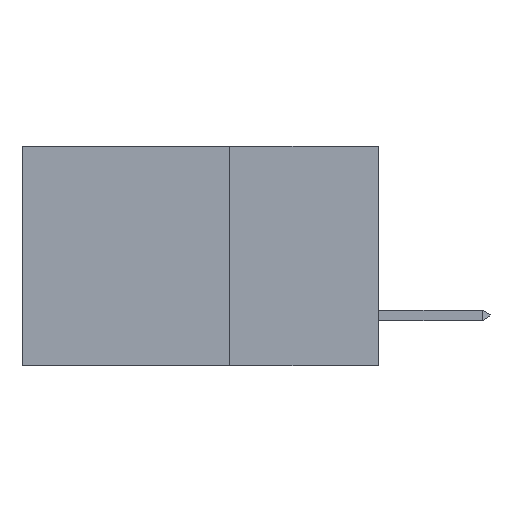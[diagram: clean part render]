
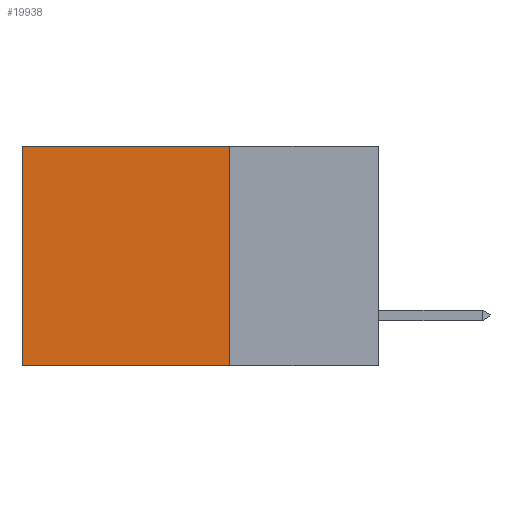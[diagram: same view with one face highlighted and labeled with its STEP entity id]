
A CAD part, left-side view. The second image highlights one B-rep face of the part: STEP entity #19938.
In plain terms, the highlighted planar face has unit normal (-1, 0, 0).
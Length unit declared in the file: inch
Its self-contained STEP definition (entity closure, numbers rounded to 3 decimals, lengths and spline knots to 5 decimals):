
#2656 = CARTESIAN_POINT ( 'NONE',  ( 0.2615, 0.25, -0.37 ) ) ;
#3022 = ORIENTED_EDGE ( 'NONE', *, *, #3099, .T. ) ;
#3099 = EDGE_CURVE ( 'NONE', #11433, #8185, #10697, .T. ) ;
#3180 = ORIENTED_EDGE ( 'NONE', *, *, #11354, .F. ) ;
#4965 = CARTESIAN_POINT ( 'NONE',  ( 0.2615, 0.6, 0. ) ) ;
#5666 = DIRECTION ( 'NONE',  ( 0., 1., 0. ) ) ;
#6414 = VECTOR ( 'NONE', #16395, 39.37008 ) ;
#6735 = VECTOR ( 'NONE', #21757, 39.37008 ) ;
#8139 = EDGE_CURVE ( 'NONE', #8185, #10181, #9805, .T. ) ;
#8185 = VERTEX_POINT ( 'NONE', #4965 ) ;
#9715 = DIRECTION ( 'NONE',  ( 1., 0., 0. ) ) ;
#9805 = LINE ( 'NONE', #16778, #13571 ) ;
#10181 = VERTEX_POINT ( 'NONE', #18547 ) ;
#10594 = CARTESIAN_POINT ( 'NONE',  ( 0.2615, 0.25, 0. ) ) ;
#10685 = VECTOR ( 'NONE', #5666, 39.37008 ) ;
#10697 = LINE ( 'NONE', #10594, #10685 ) ;
#11214 = CARTESIAN_POINT ( 'NONE',  ( 0.2615, 0.25, 0. ) ) ;
#11354 = EDGE_CURVE ( 'NONE', #17194, #10181, #16244, .T. ) ;
#11433 = VERTEX_POINT ( 'NONE', #11214 ) ;
#12686 = CARTESIAN_POINT ( 'NONE',  ( 0.2615, 0.25, -0.37 ) ) ;
#12820 = LINE ( 'NONE', #2656, #6414 ) ;
#13531 = CARTESIAN_POINT ( 'NONE',  ( 0.2615, 0.25, -0.37 ) ) ;
#13571 = VECTOR ( 'NONE', #20457, 39.37008 ) ;
#14750 = PLANE ( 'NONE',  #19535 ) ;
#15087 = CARTESIAN_POINT ( 'NONE',  ( 0.2615, 0.25, -0.37 ) ) ;
#15461 = EDGE_LOOP ( 'NONE', ( #20952, #3180, #16371, #3022 ) ) ;
#16244 = LINE ( 'NONE', #12686, #6735 ) ;
#16371 = ORIENTED_EDGE ( 'NONE', *, *, #21071, .F. ) ;
#16395 = DIRECTION ( 'NONE',  ( 0., 0., -1. ) ) ;
#16778 = CARTESIAN_POINT ( 'NONE',  ( 0.2615, 0.6, -0.37 ) ) ;
#17194 = VERTEX_POINT ( 'NONE', #13531 ) ;
#18204 = DIRECTION ( 'NONE',  ( 0., 0., -1. ) ) ;
#18422 = FACE_OUTER_BOUND ( 'NONE', #15461, .T. ) ;
#18547 = CARTESIAN_POINT ( 'NONE',  ( 0.2615, 0.6, -0.37 ) ) ;
#19535 = AXIS2_PLACEMENT_3D ( 'NONE', #15087, #9715, #18204 ) ;
#19938 = ADVANCED_FACE ( 'NONE', ( #18422 ), #14750, .F. ) ;
#20457 = DIRECTION ( 'NONE',  ( 0., 0., -1. ) ) ;
#20952 = ORIENTED_EDGE ( 'NONE', *, *, #8139, .T. ) ;
#21071 = EDGE_CURVE ( 'NONE', #11433, #17194, #12820, .T. ) ;
#21757 = DIRECTION ( 'NONE',  ( 0., 1., 0. ) ) ;
